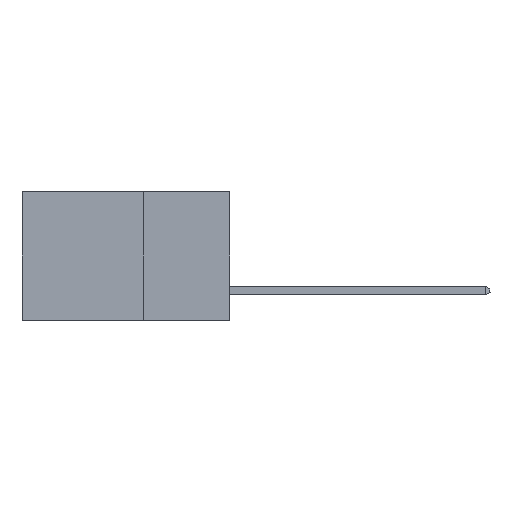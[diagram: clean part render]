
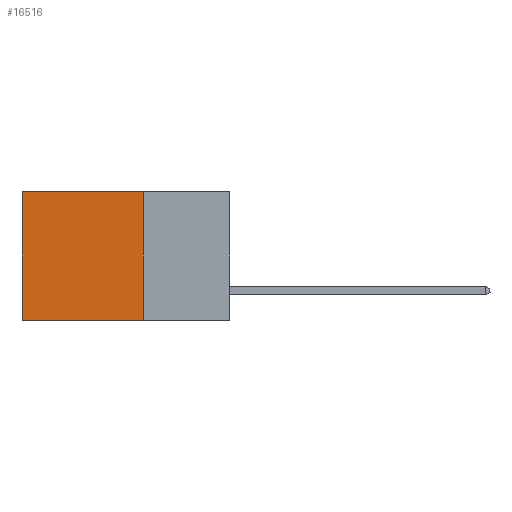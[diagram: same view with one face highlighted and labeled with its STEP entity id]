
A CAD part, left-side view. The second image highlights one B-rep face of the part: STEP entity #16516.
In plain terms, the highlighted planar face has unit normal (-1, 0, 0).
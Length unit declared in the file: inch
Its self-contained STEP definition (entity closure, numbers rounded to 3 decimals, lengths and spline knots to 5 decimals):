
#66 = DIRECTION ( 'NONE',  ( 1., 0., 0. ) ) ;
#981 = CARTESIAN_POINT ( 'NONE',  ( 0.298, 0.25, 0. ) ) ;
#1161 = LINE ( 'NONE', #24123, #6460 ) ;
#1632 = VERTEX_POINT ( 'NONE', #7878 ) ;
#1791 = EDGE_CURVE ( 'NONE', #10250, #27832, #1161, .T. ) ;
#2382 = LINE ( 'NONE', #21886, #25754 ) ;
#6075 = LINE ( 'NONE', #15231, #23776 ) ;
#6392 = CARTESIAN_POINT ( 'NONE',  ( 0.298, 0.25, -0.37 ) ) ;
#6460 = VECTOR ( 'NONE', #12457, 39.37008 ) ;
#7878 = CARTESIAN_POINT ( 'NONE',  ( 0.298, 0.6, 0. ) ) ;
#8728 = EDGE_CURVE ( 'NONE', #27660, #1632, #10451, .T. ) ;
#10250 = VERTEX_POINT ( 'NONE', #6392 ) ;
#10451 = LINE ( 'NONE', #981, #12233 ) ;
#10600 = EDGE_CURVE ( 'NONE', #1632, #27832, #6075, .T. ) ;
#12233 = VECTOR ( 'NONE', #21649, 39.37008 ) ;
#12457 = DIRECTION ( 'NONE',  ( 0., 1., 0. ) ) ;
#15128 = CARTESIAN_POINT ( 'NONE',  ( 0.298, 0.25, 0. ) ) ;
#15231 = CARTESIAN_POINT ( 'NONE',  ( 0.298, 0.6, 0. ) ) ;
#16516 = ADVANCED_FACE ( 'NONE', ( #25729 ), #20431, .F. ) ;
#16879 = ORIENTED_EDGE ( 'NONE', *, *, #10600, .T. ) ;
#17345 = DIRECTION ( 'NONE',  ( 0., 0., -1. ) ) ;
#20431 = PLANE ( 'NONE',  #22385 ) ;
#21649 = DIRECTION ( 'NONE',  ( 0., 1., 0. ) ) ;
#21886 = CARTESIAN_POINT ( 'NONE',  ( 0.298, 0.25, 0. ) ) ;
#21919 = DIRECTION ( 'NONE',  ( 0., 0., -1. ) ) ;
#21949 = EDGE_LOOP ( 'NONE', ( #16879, #24762, #29129, #26518 ) ) ;
#22272 = CARTESIAN_POINT ( 'NONE',  ( 0.298, 0.6, -0.37 ) ) ;
#22385 = AXIS2_PLACEMENT_3D ( 'NONE', #27382, #66, #27079 ) ;
#23776 = VECTOR ( 'NONE', #21919, 39.37008 ) ;
#24123 = CARTESIAN_POINT ( 'NONE',  ( 0.298, 0.25, -0.37 ) ) ;
#24762 = ORIENTED_EDGE ( 'NONE', *, *, #1791, .F. ) ;
#25729 = FACE_OUTER_BOUND ( 'NONE', #21949, .T. ) ;
#25754 = VECTOR ( 'NONE', #17345, 39.37008 ) ;
#26518 = ORIENTED_EDGE ( 'NONE', *, *, #8728, .T. ) ;
#27079 = DIRECTION ( 'NONE',  ( 0., 0., -1. ) ) ;
#27382 = CARTESIAN_POINT ( 'NONE',  ( 0.298, 0.25, 0. ) ) ;
#27660 = VERTEX_POINT ( 'NONE', #15128 ) ;
#27832 = VERTEX_POINT ( 'NONE', #22272 ) ;
#28981 = EDGE_CURVE ( 'NONE', #27660, #10250, #2382, .T. ) ;
#29129 = ORIENTED_EDGE ( 'NONE', *, *, #28981, .F. ) ;
